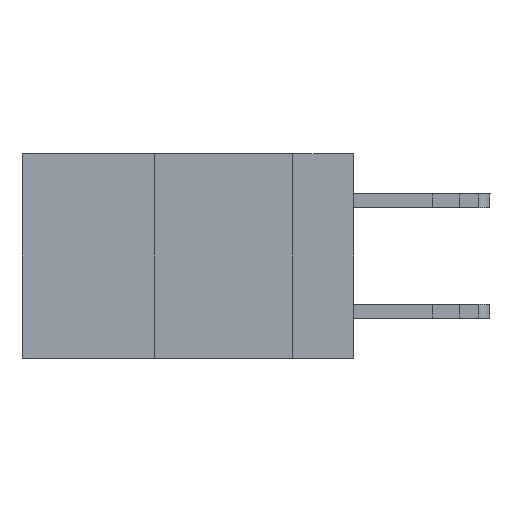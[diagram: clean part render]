
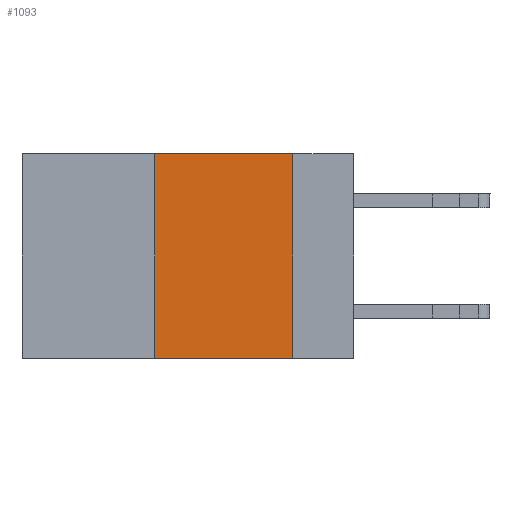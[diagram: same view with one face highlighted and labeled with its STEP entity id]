
A CAD part, left-side view. The second image highlights one B-rep face of the part: STEP entity #1093.
In plain terms, the highlighted planar face has unit normal (-1, 0, 0).
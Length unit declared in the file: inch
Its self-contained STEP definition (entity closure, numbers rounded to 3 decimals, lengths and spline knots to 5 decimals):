
#385 = DIRECTION ( 'NONE',  ( 0., 0., -1. ) ) ;
#510 = CARTESIAN_POINT ( 'NONE',  ( 0., 0.36, 0. ) ) ;
#518 = LINE ( 'NONE', #19354, #5719 ) ;
#582 = VECTOR ( 'NONE', #18738, 39.37008 ) ;
#661 = LINE ( 'NONE', #510, #2872 ) ;
#1093 = ADVANCED_FACE ( 'NONE', ( #22104 ), #21569, .F. ) ;
#1164 = EDGE_CURVE ( 'NONE', #4047, #6101, #518, .T. ) ;
#1280 = CARTESIAN_POINT ( 'NONE',  ( 0., 0.6, -0.37 ) ) ;
#2855 = EDGE_LOOP ( 'NONE', ( #11237, #12664, #21458, #13855 ) ) ;
#2872 = VECTOR ( 'NONE', #12745, 39.37008 ) ;
#3609 = LINE ( 'NONE', #1280, #582 ) ;
#3687 = VERTEX_POINT ( 'NONE', #11012 ) ;
#4047 = VERTEX_POINT ( 'NONE', #17262 ) ;
#4502 = CARTESIAN_POINT ( 'NONE',  ( 0., 0.36, -0.37 ) ) ;
#4669 = EDGE_CURVE ( 'NONE', #9357, #3687, #3609, .T. ) ;
#5593 = DIRECTION ( 'NONE',  ( 0., -1., 0. ) ) ;
#5719 = VECTOR ( 'NONE', #5593, 39.37008 ) ;
#6101 = VERTEX_POINT ( 'NONE', #17412 ) ;
#7817 = LINE ( 'NONE', #15694, #8378 ) ;
#8378 = VECTOR ( 'NONE', #385, 39.37008 ) ;
#8793 = CARTESIAN_POINT ( 'NONE',  ( 0., 0.6, 0. ) ) ;
#9304 = EDGE_CURVE ( 'NONE', #9357, #4047, #661, .T. ) ;
#9357 = VERTEX_POINT ( 'NONE', #4502 ) ;
#10136 = AXIS2_PLACEMENT_3D ( 'NONE', #8793, #17592, #16914 ) ;
#11012 = CARTESIAN_POINT ( 'NONE',  ( 0., 0.11, -0.37 ) ) ;
#11237 = ORIENTED_EDGE ( 'NONE', *, *, #20021, .F. ) ;
#12664 = ORIENTED_EDGE ( 'NONE', *, *, #1164, .F. ) ;
#12745 = DIRECTION ( 'NONE',  ( 0., 0., 1. ) ) ;
#13855 = ORIENTED_EDGE ( 'NONE', *, *, #4669, .T. ) ;
#15694 = CARTESIAN_POINT ( 'NONE',  ( 0., 0.11, 0. ) ) ;
#16914 = DIRECTION ( 'NONE',  ( 0., 0., -1. ) ) ;
#17262 = CARTESIAN_POINT ( 'NONE',  ( 0., 0.36, 0. ) ) ;
#17412 = CARTESIAN_POINT ( 'NONE',  ( 0., 0.11, 0. ) ) ;
#17592 = DIRECTION ( 'NONE',  ( 1., 0., 0. ) ) ;
#18738 = DIRECTION ( 'NONE',  ( 0., -1., 0. ) ) ;
#19354 = CARTESIAN_POINT ( 'NONE',  ( 0., 0.6, 0. ) ) ;
#20021 = EDGE_CURVE ( 'NONE', #6101, #3687, #7817, .T. ) ;
#21458 = ORIENTED_EDGE ( 'NONE', *, *, #9304, .F. ) ;
#21569 = PLANE ( 'NONE',  #10136 ) ;
#22104 = FACE_OUTER_BOUND ( 'NONE', #2855, .T. ) ;
